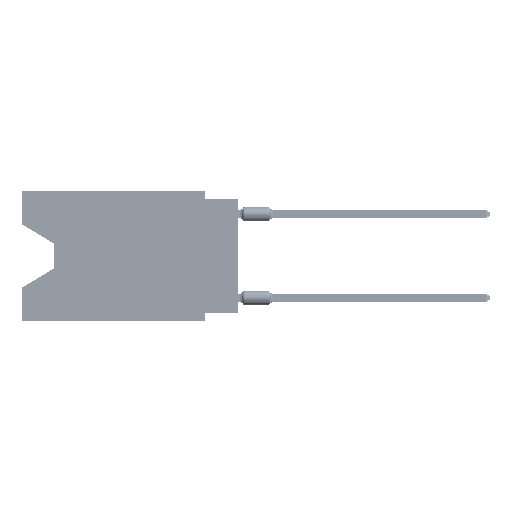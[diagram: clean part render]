
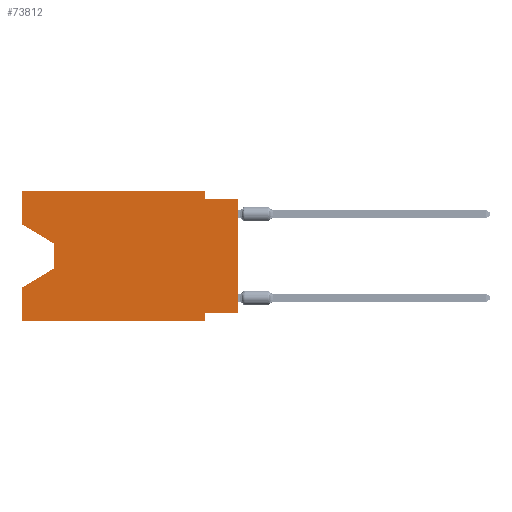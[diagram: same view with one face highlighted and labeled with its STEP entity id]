
A CAD part, left-side view. The second image highlights one B-rep face of the part: STEP entity #73812.
In plain terms, the highlighted planar face has unit normal (-1, 0, 0).
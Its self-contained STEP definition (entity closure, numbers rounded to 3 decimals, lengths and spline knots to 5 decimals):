
#596 = ORIENTED_EDGE ( 'NONE', *, *, #48889, .F. ) ;
#1150 = CARTESIAN_POINT ( 'NONE',  ( 0., 0., -0.365 ) ) ;
#1314 = CARTESIAN_POINT ( 'NONE',  ( 0., 0.645, -0.10025 ) ) ;
#1589 = CARTESIAN_POINT ( 'NONE',  ( 0., 0.645, 0. ) ) ;
#1602 = VERTEX_POINT ( 'NONE', #29639 ) ;
#3676 = DIRECTION ( 'NONE',  ( 0., 1., 0. ) ) ;
#4506 = DIRECTION ( 'NONE',  ( 0., 0., -1. ) ) ;
#5357 = CARTESIAN_POINT ( 'NONE',  ( 0., 0.645, -0.10025 ) ) ;
#5789 = DIRECTION ( 'NONE',  ( 0., -0.855, -0.519 ) ) ;
#5848 = LINE ( 'NONE', #18263, #47983 ) ;
#8889 = VECTOR ( 'NONE', #28547, 39.37008 ) ;
#9089 = LINE ( 'NONE', #1589, #8889 ) ;
#9599 = VECTOR ( 'NONE', #67102, 39.37008 ) ;
#10147 = EDGE_CURVE ( 'NONE', #13129, #50811, #51184, .T. ) ;
#12543 = VERTEX_POINT ( 'NONE', #42699 ) ;
#13129 = VERTEX_POINT ( 'NONE', #83651 ) ;
#14477 = ORIENTED_EDGE ( 'NONE', *, *, #52214, .F. ) ;
#14581 = VERTEX_POINT ( 'NONE', #30908 ) ;
#15336 = ORIENTED_EDGE ( 'NONE', *, *, #18144, .T. ) ;
#16155 = VECTOR ( 'NONE', #55506, 39.37008 ) ;
#16445 = VERTEX_POINT ( 'NONE', #1150 ) ;
#16948 = LINE ( 'NONE', #72518, #85180 ) ;
#17767 = LINE ( 'NONE', #5357, #25711 ) ;
#18144 = EDGE_CURVE ( 'NONE', #37173, #30637, #17767, .T. ) ;
#18263 = CARTESIAN_POINT ( 'NONE',  ( 0., 0.645, 0. ) ) ;
#18821 = VECTOR ( 'NONE', #43924, 39.37008 ) ;
#19204 = EDGE_CURVE ( 'NONE', #1602, #14581, #9089, .T. ) ;
#19816 = LINE ( 'NONE', #53367, #18821 ) ;
#21157 = VECTOR ( 'NONE', #4506, 39.37008 ) ;
#21260 = DIRECTION ( 'NONE',  ( 0., 0., 1. ) ) ;
#23671 = VECTOR ( 'NONE', #21260, 39.37008 ) ;
#25089 = CARTESIAN_POINT ( 'NONE',  ( 0., 0.55, -0.158 ) ) ;
#25711 = VECTOR ( 'NONE', #5789, 39.37008 ) ;
#26051 = LINE ( 'NONE', #77428, #9599 ) ;
#26508 = PLANE ( 'NONE',  #77875 ) ;
#28547 = DIRECTION ( 'NONE',  ( 0., -1., 0. ) ) ;
#29633 = LINE ( 'NONE', #68070, #23671 ) ;
#29639 = CARTESIAN_POINT ( 'NONE',  ( 0., 0.645, 0. ) ) ;
#30637 = VERTEX_POINT ( 'NONE', #25089 ) ;
#30908 = CARTESIAN_POINT ( 'NONE',  ( 0., 0.1, 0. ) ) ;
#31052 = EDGE_CURVE ( 'NONE', #14581, #63986, #76239, .T. ) ;
#32496 = VECTOR ( 'NONE', #74162, 39.37008 ) ;
#32769 = DIRECTION ( 'NONE',  ( 0., 0., 1. ) ) ;
#37173 = VERTEX_POINT ( 'NONE', #1314 ) ;
#39353 = LINE ( 'NONE', #64990, #21157 ) ;
#40624 = VERTEX_POINT ( 'NONE', #69717 ) ;
#41010 = VECTOR ( 'NONE', #63134, 39.37008 ) ;
#41322 = ORIENTED_EDGE ( 'NONE', *, *, #68284, .T. ) ;
#41452 = EDGE_CURVE ( 'NONE', #63986, #40624, #26051, .T. ) ;
#42011 = CARTESIAN_POINT ( 'NONE',  ( 0., 0.1, -0.365 ) ) ;
#42699 = CARTESIAN_POINT ( 'NONE',  ( 0., 0.645, -0.39 ) ) ;
#43598 = EDGE_CURVE ( 'NONE', #30637, #13129, #79914, .T. ) ;
#43735 = CARTESIAN_POINT ( 'NONE',  ( 0., 0.645, -0.28975 ) ) ;
#43760 = EDGE_CURVE ( 'NONE', #12543, #50811, #49859, .T. ) ;
#43924 = DIRECTION ( 'NONE',  ( 0., -1., 0. ) ) ;
#46037 = EDGE_CURVE ( 'NONE', #16445, #40624, #29633, .T. ) ;
#46777 = EDGE_LOOP ( 'NONE', ( #15336, #83836, #66060, #84464, #41322, #76600, #14477, #82606, #61627, #57388, #67949, #596 ) ) ;
#47248 = DIRECTION ( 'NONE',  ( 1., 0., 0. ) ) ;
#47983 = VECTOR ( 'NONE', #32769, 39.37008 ) ;
#48889 = EDGE_CURVE ( 'NONE', #37173, #1602, #5848, .T. ) ;
#49859 = LINE ( 'NONE', #76774, #77702 ) ;
#50811 = VERTEX_POINT ( 'NONE', #43735 ) ;
#51184 = LINE ( 'NONE', #70619, #41010 ) ;
#52214 = EDGE_CURVE ( 'NONE', #16445, #78158, #16948, .T. ) ;
#53367 = CARTESIAN_POINT ( 'NONE',  ( 0., 0.645, -0.39 ) ) ;
#55445 = CARTESIAN_POINT ( 'NONE',  ( 0., 0.1, -0.025 ) ) ;
#55506 = DIRECTION ( 'NONE',  ( 0., 0., -1. ) ) ;
#57388 = ORIENTED_EDGE ( 'NONE', *, *, #31052, .F. ) ;
#59790 = VERTEX_POINT ( 'NONE', #60204 ) ;
#60040 = CARTESIAN_POINT ( 'NONE',  ( 0., 0.645, 0. ) ) ;
#60204 = CARTESIAN_POINT ( 'NONE',  ( 0., 0.1, -0.39 ) ) ;
#61353 = CARTESIAN_POINT ( 'NONE',  ( 0., 0.55, -0.158 ) ) ;
#61361 = DIRECTION ( 'NONE',  ( 0., 0., -1. ) ) ;
#61627 = ORIENTED_EDGE ( 'NONE', *, *, #41452, .F. ) ;
#63134 = DIRECTION ( 'NONE',  ( 0., 0.855, -0.519 ) ) ;
#63986 = VERTEX_POINT ( 'NONE', #55445 ) ;
#64781 = EDGE_CURVE ( 'NONE', #78158, #59790, #39353, .T. ) ;
#64990 = CARTESIAN_POINT ( 'NONE',  ( 0., 0.1, -0.39 ) ) ;
#66060 = ORIENTED_EDGE ( 'NONE', *, *, #10147, .T. ) ;
#66675 = FACE_OUTER_BOUND ( 'NONE', #46777, .T. ) ;
#67102 = DIRECTION ( 'NONE',  ( 0., -1., 0. ) ) ;
#67949 = ORIENTED_EDGE ( 'NONE', *, *, #19204, .F. ) ;
#68070 = CARTESIAN_POINT ( 'NONE',  ( 0., 0., 0. ) ) ;
#68284 = EDGE_CURVE ( 'NONE', #12543, #59790, #19816, .T. ) ;
#69717 = CARTESIAN_POINT ( 'NONE',  ( 0., 0., -0.025 ) ) ;
#70619 = CARTESIAN_POINT ( 'NONE',  ( 0., 0.55, -0.232 ) ) ;
#72518 = CARTESIAN_POINT ( 'NONE',  ( 0., 0., -0.365 ) ) ;
#73812 = ADVANCED_FACE ( 'NONE', ( #66675 ), #26508, .F. ) ;
#74162 = DIRECTION ( 'NONE',  ( 0., 0., -1. ) ) ;
#76239 = LINE ( 'NONE', #82863, #16155 ) ;
#76600 = ORIENTED_EDGE ( 'NONE', *, *, #64781, .F. ) ;
#76774 = CARTESIAN_POINT ( 'NONE',  ( 0., 0.645, 0. ) ) ;
#77428 = CARTESIAN_POINT ( 'NONE',  ( 0., 0., -0.025 ) ) ;
#77702 = VECTOR ( 'NONE', #83832, 39.37008 ) ;
#77875 = AXIS2_PLACEMENT_3D ( 'NONE', #60040, #47248, #61361 ) ;
#78158 = VERTEX_POINT ( 'NONE', #42011 ) ;
#79914 = LINE ( 'NONE', #61353, #32496 ) ;
#82606 = ORIENTED_EDGE ( 'NONE', *, *, #46037, .T. ) ;
#82863 = CARTESIAN_POINT ( 'NONE',  ( 0., 0.1, 0. ) ) ;
#83651 = CARTESIAN_POINT ( 'NONE',  ( 0., 0.55, -0.232 ) ) ;
#83832 = DIRECTION ( 'NONE',  ( 0., 0., 1. ) ) ;
#83836 = ORIENTED_EDGE ( 'NONE', *, *, #43598, .T. ) ;
#84464 = ORIENTED_EDGE ( 'NONE', *, *, #43760, .F. ) ;
#85180 = VECTOR ( 'NONE', #3676, 39.37008 ) ;
